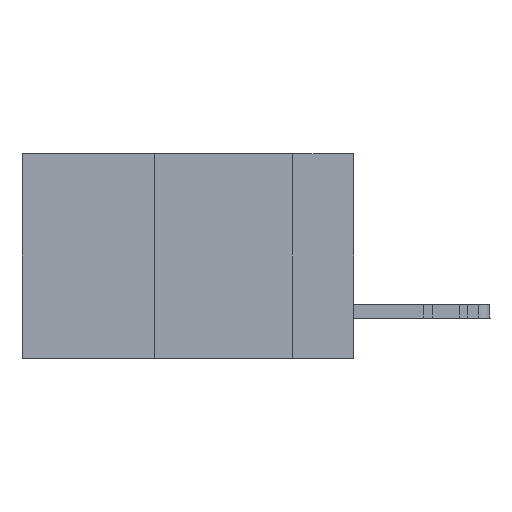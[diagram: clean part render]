
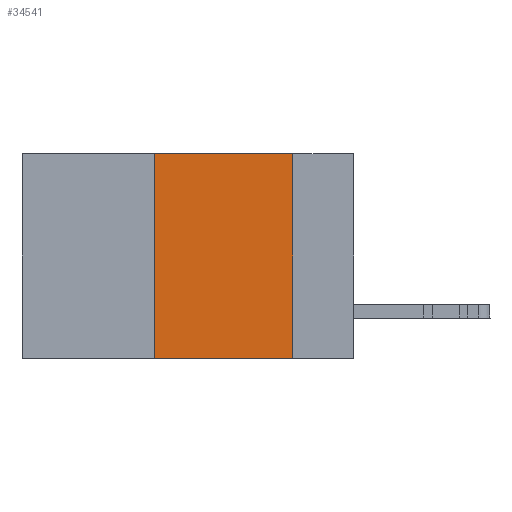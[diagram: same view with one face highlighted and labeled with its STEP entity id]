
A CAD part, left-side view. The second image highlights one B-rep face of the part: STEP entity #34541.
In plain terms, the highlighted planar face has unit normal (-1, 0, 0).
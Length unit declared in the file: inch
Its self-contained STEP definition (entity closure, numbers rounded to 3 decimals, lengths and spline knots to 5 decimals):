
#79 = CARTESIAN_POINT ( 'NONE',  ( 0., 0.11, 0. ) ) ;
#150 = CARTESIAN_POINT ( 'NONE',  ( 0., 0.6, 0. ) ) ;
#1369 = VERTEX_POINT ( 'NONE', #39176 ) ;
#2439 = ORIENTED_EDGE ( 'NONE', *, *, #40904, .F. ) ;
#3827 = LINE ( 'NONE', #150, #13934 ) ;
#5882 = EDGE_CURVE ( 'NONE', #33574, #29172, #14596, .T. ) ;
#7263 = LINE ( 'NONE', #79, #36963 ) ;
#9233 = CARTESIAN_POINT ( 'NONE',  ( 0., 0.36, -0.37 ) ) ;
#9349 = DIRECTION ( 'NONE',  ( 0., -1., 0. ) ) ;
#11133 = DIRECTION ( 'NONE',  ( 0., -1., 0. ) ) ;
#13934 = VECTOR ( 'NONE', #11133, 39.37008 ) ;
#14596 = LINE ( 'NONE', #30819, #33138 ) ;
#14899 = DIRECTION ( 'NONE',  ( 0., 0., -1. ) ) ;
#15727 = CARTESIAN_POINT ( 'NONE',  ( 0., 0.36, 0. ) ) ;
#17213 = EDGE_LOOP ( 'NONE', ( #24770, #2439, #21302, #40005 ) ) ;
#21302 = ORIENTED_EDGE ( 'NONE', *, *, #32645, .F. ) ;
#22156 = DIRECTION ( 'NONE',  ( 0., 0., -1. ) ) ;
#24770 = ORIENTED_EDGE ( 'NONE', *, *, #29073, .F. ) ;
#26246 = CARTESIAN_POINT ( 'NONE',  ( 0., 0.11, -0.37 ) ) ;
#26745 = FACE_OUTER_BOUND ( 'NONE', #17213, .T. ) ;
#26777 = VERTEX_POINT ( 'NONE', #15727 ) ;
#26944 = LINE ( 'NONE', #35877, #43207 ) ;
#28837 = CARTESIAN_POINT ( 'NONE',  ( 0., 0.6, 0. ) ) ;
#29073 = EDGE_CURVE ( 'NONE', #1369, #29172, #7263, .T. ) ;
#29145 = PLANE ( 'NONE',  #30743 ) ;
#29172 = VERTEX_POINT ( 'NONE', #26246 ) ;
#30743 = AXIS2_PLACEMENT_3D ( 'NONE', #28837, #43428, #14899 ) ;
#30819 = CARTESIAN_POINT ( 'NONE',  ( 0., 0.6, -0.37 ) ) ;
#32033 = DIRECTION ( 'NONE',  ( 0., 0., 1. ) ) ;
#32645 = EDGE_CURVE ( 'NONE', #33574, #26777, #26944, .T. ) ;
#33138 = VECTOR ( 'NONE', #9349, 39.37008 ) ;
#33574 = VERTEX_POINT ( 'NONE', #9233 ) ;
#34541 = ADVANCED_FACE ( 'NONE', ( #26745 ), #29145, .F. ) ;
#35877 = CARTESIAN_POINT ( 'NONE',  ( 0., 0.36, 0. ) ) ;
#36963 = VECTOR ( 'NONE', #22156, 39.37008 ) ;
#39176 = CARTESIAN_POINT ( 'NONE',  ( 0., 0.11, 0. ) ) ;
#40005 = ORIENTED_EDGE ( 'NONE', *, *, #5882, .T. ) ;
#40904 = EDGE_CURVE ( 'NONE', #26777, #1369, #3827, .T. ) ;
#43207 = VECTOR ( 'NONE', #32033, 39.37008 ) ;
#43428 = DIRECTION ( 'NONE',  ( 1., 0., 0. ) ) ;
